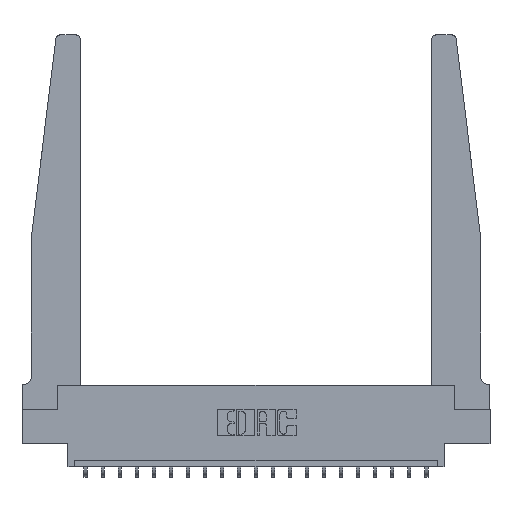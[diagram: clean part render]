
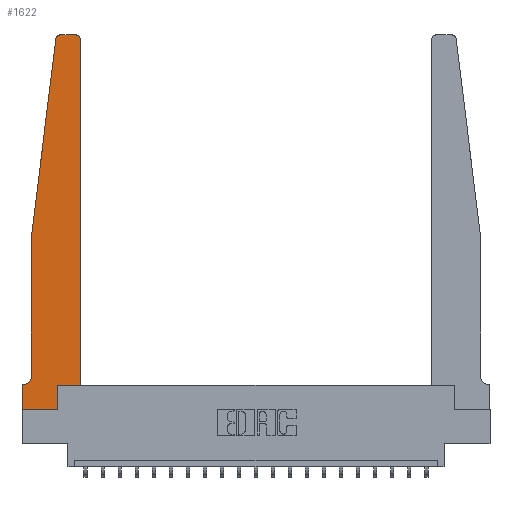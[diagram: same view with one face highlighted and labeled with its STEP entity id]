
A CAD part, top view. The second image highlights one B-rep face of the part: STEP entity #1622.
In plain terms, the highlighted planar face has unit normal (0, 0, 1).
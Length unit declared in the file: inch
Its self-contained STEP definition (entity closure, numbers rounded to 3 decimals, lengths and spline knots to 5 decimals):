
#86 = ORIENTED_EDGE ( 'NONE', *, *, #8515, .T. ) ;
#121 = CARTESIAN_POINT ( 'NONE',  ( 0., 0., 0.37 ) ) ;
#138 = ORIENTED_EDGE ( 'NONE', *, *, #15261, .T. ) ;
#257 = CARTESIAN_POINT ( 'NONE',  ( 0., 0., 0.37 ) ) ;
#797 = CARTESIAN_POINT ( 'NONE',  ( 0., 0., 0.37 ) ) ;
#815 = DIRECTION ( 'NONE',  ( -0.122, -0.992, 0. ) ) ;
#926 = CARTESIAN_POINT ( 'NONE',  ( 0.065, 1.25, 0.37 ) ) ;
#1312 = LINE ( 'NONE', #11413, #16584 ) ;
#1355 = VERTEX_POINT ( 'NONE', #17717 ) ;
#1390 = CARTESIAN_POINT ( 'NONE',  ( 0.015, 0.1875, 0.37 ) ) ;
#1622 = ADVANCED_FACE ( 'NONE', ( #16317 ), #19539, .T. ) ;
#1995 = VECTOR ( 'NONE', #9545, 39.37008 ) ;
#2030 = LINE ( 'NONE', #8608, #8117 ) ;
#2156 = VERTEX_POINT ( 'NONE', #10457 ) ;
#2339 = VERTEX_POINT ( 'NONE', #12402 ) ;
#2403 = EDGE_CURVE ( 'NONE', #16241, #1355, #1312, .T. ) ;
#2952 = EDGE_CURVE ( 'NONE', #19691, #5746, #2030, .T. ) ;
#3108 = VERTEX_POINT ( 'NONE', #16983 ) ;
#3351 = ORIENTED_EDGE ( 'NONE', *, *, #17008, .T. ) ;
#3553 = EDGE_CURVE ( 'NONE', #1355, #17381, #8109, .T. ) ;
#3592 = CARTESIAN_POINT ( 'NONE',  ( 0.27653, 2.75, 0.37 ) ) ;
#3903 = ORIENTED_EDGE ( 'NONE', *, *, #17429, .T. ) ;
#4144 = DIRECTION ( 'NONE',  ( 1., 0., 0. ) ) ;
#4485 = EDGE_CURVE ( 'NONE', #20452, #2156, #11691, .T. ) ;
#4582 = DIRECTION ( 'NONE',  ( 0., 0., -1. ) ) ;
#4667 = DIRECTION ( 'NONE',  ( 0., -1., 0. ) ) ;
#4692 = ORIENTED_EDGE ( 'NONE', *, *, #2403, .T. ) ;
#4798 = EDGE_CURVE ( 'NONE', #14378, #2339, #19421, .T. ) ;
#4809 = CARTESIAN_POINT ( 'NONE',  ( 0., 0.1875, 0.37 ) ) ;
#5261 = CARTESIAN_POINT ( 'NONE',  ( 0.2605, 0., 0.37 ) ) ;
#5374 = DIRECTION ( 'NONE',  ( 1., 0., 0. ) ) ;
#5746 = VERTEX_POINT ( 'NONE', #7887 ) ;
#7506 = LINE ( 'NONE', #926, #7927 ) ;
#7887 = CARTESIAN_POINT ( 'NONE',  ( 0.2605, 0.18, 0.37 ) ) ;
#7922 = CARTESIAN_POINT ( 'NONE',  ( 0.015, 0.2375, 0.37 ) ) ;
#7927 = VECTOR ( 'NONE', #815, 39.37008 ) ;
#8109 = LINE ( 'NONE', #121, #18549 ) ;
#8117 = VECTOR ( 'NONE', #8704, 39.37008 ) ;
#8212 = DIRECTION ( 'NONE',  ( -1., 0., 0. ) ) ;
#8515 = EDGE_CURVE ( 'NONE', #12634, #16777, #20770, .T. ) ;
#8608 = CARTESIAN_POINT ( 'NONE',  ( 0.2605, 0.18, 0.37 ) ) ;
#8704 = DIRECTION ( 'NONE',  ( 0., 1., 0. ) ) ;
#8767 = DIRECTION ( 'NONE',  ( 0., 0., 1. ) ) ;
#8903 = ORIENTED_EDGE ( 'NONE', *, *, #4798, .T. ) ;
#9539 = ORIENTED_EDGE ( 'NONE', *, *, #13835, .T. ) ;
#9545 = DIRECTION ( 'NONE',  ( 0., 1., 0. ) ) ;
#10457 = CARTESIAN_POINT ( 'NONE',  ( 0.065, 0.2375, 0.37 ) ) ;
#10660 = VECTOR ( 'NONE', #18340, 39.37008 ) ;
#11119 = DIRECTION ( 'NONE',  ( 0., 0., 1. ) ) ;
#11406 = CARTESIAN_POINT ( 'NONE',  ( 0.065, 1.25, 0.37 ) ) ;
#11413 = CARTESIAN_POINT ( 'NONE',  ( 0.065, 0.1875, 0.37 ) ) ;
#11642 = AXIS2_PLACEMENT_3D ( 'NONE', #12601, #21010, #19383 ) ;
#11691 = LINE ( 'NONE', #18465, #15013 ) ;
#11775 = LINE ( 'NONE', #17915, #10660 ) ;
#12402 = CARTESIAN_POINT ( 'NONE',  ( 0.425, 2.72, 0.37 ) ) ;
#12558 = CARTESIAN_POINT ( 'NONE',  ( 0.24675, 2.72367, 0.37 ) ) ;
#12600 = ORIENTED_EDGE ( 'NONE', *, *, #2952, .T. ) ;
#12601 = CARTESIAN_POINT ( 'NONE',  ( 0.395, 2.72, 0.37 ) ) ;
#12634 = VERTEX_POINT ( 'NONE', #3592 ) ;
#12652 = CIRCLE ( 'NONE', #17487, 0.05 ) ;
#12858 = CARTESIAN_POINT ( 'NONE',  ( 0.425, 0.18, 0.37 ) ) ;
#13240 = ORIENTED_EDGE ( 'NONE', *, *, #16314, .T. ) ;
#13732 = AXIS2_PLACEMENT_3D ( 'NONE', #4809, #8767, #18668 ) ;
#13835 = EDGE_CURVE ( 'NONE', #17381, #19691, #18769, .T. ) ;
#14378 = VERTEX_POINT ( 'NONE', #19277 ) ;
#15013 = VECTOR ( 'NONE', #19873, 39.37008 ) ;
#15261 = EDGE_CURVE ( 'NONE', #2156, #16241, #12652, .T. ) ;
#15637 = EDGE_CURVE ( 'NONE', #2339, #3108, #18181, .T. ) ;
#16073 = DIRECTION ( 'NONE',  ( -1., 0., 0. ) ) ;
#16241 = VERTEX_POINT ( 'NONE', #1390 ) ;
#16314 = EDGE_CURVE ( 'NONE', #5746, #14378, #20417, .T. ) ;
#16317 = FACE_OUTER_BOUND ( 'NONE', #19368, .T. ) ;
#16506 = CARTESIAN_POINT ( 'NONE',  ( 0.27653, 2.72, 0.37 ) ) ;
#16584 = VECTOR ( 'NONE', #8212, 39.37008 ) ;
#16772 = CARTESIAN_POINT ( 'NONE',  ( 0.425, 0.18, 0.37 ) ) ;
#16777 = VERTEX_POINT ( 'NONE', #12558 ) ;
#16983 = CARTESIAN_POINT ( 'NONE',  ( 0.395, 2.75, 0.37 ) ) ;
#17008 = EDGE_CURVE ( 'NONE', #16777, #20452, #7506, .T. ) ;
#17381 = VERTEX_POINT ( 'NONE', #257 ) ;
#17429 = EDGE_CURVE ( 'NONE', #3108, #12634, #11775, .T. ) ;
#17453 = ORIENTED_EDGE ( 'NONE', *, *, #4485, .T. ) ;
#17487 = AXIS2_PLACEMENT_3D ( 'NONE', #7922, #4582, #16073 ) ;
#17519 = VECTOR ( 'NONE', #5374, 39.37008 ) ;
#17717 = CARTESIAN_POINT ( 'NONE',  ( 0., 0.1875, 0.37 ) ) ;
#17915 = CARTESIAN_POINT ( 'NONE',  ( 0.25, 2.75, 0.37 ) ) ;
#18181 = CIRCLE ( 'NONE', #11642, 0.03 ) ;
#18340 = DIRECTION ( 'NONE',  ( -1., 0., 0. ) ) ;
#18465 = CARTESIAN_POINT ( 'NONE',  ( 0.065, 1.25, 0.37 ) ) ;
#18491 = ORIENTED_EDGE ( 'NONE', *, *, #3553, .T. ) ;
#18549 = VECTOR ( 'NONE', #4667, 39.37008 ) ;
#18668 = DIRECTION ( 'NONE',  ( 1., 0., 0. ) ) ;
#18769 = LINE ( 'NONE', #797, #20170 ) ;
#19277 = CARTESIAN_POINT ( 'NONE',  ( 0.425, 0.18, 0.37 ) ) ;
#19368 = EDGE_LOOP ( 'NONE', ( #3903, #86, #3351, #17453, #138, #4692, #18491, #9539, #12600, #13240, #8903, #20565 ) ) ;
#19383 = DIRECTION ( 'NONE',  ( 1., 0., 0. ) ) ;
#19421 = LINE ( 'NONE', #12858, #1995 ) ;
#19539 = PLANE ( 'NONE',  #13732 ) ;
#19691 = VERTEX_POINT ( 'NONE', #5261 ) ;
#19731 = DIRECTION ( 'NONE',  ( 1., 0., 0. ) ) ;
#19873 = DIRECTION ( 'NONE',  ( 0., -1., 0. ) ) ;
#20170 = VECTOR ( 'NONE', #4144, 39.37008 ) ;
#20417 = LINE ( 'NONE', #16772, #17519 ) ;
#20452 = VERTEX_POINT ( 'NONE', #11406 ) ;
#20565 = ORIENTED_EDGE ( 'NONE', *, *, #15637, .T. ) ;
#20770 = CIRCLE ( 'NONE', #21120, 0.03 ) ;
#21010 = DIRECTION ( 'NONE',  ( 0., 0., 1. ) ) ;
#21120 = AXIS2_PLACEMENT_3D ( 'NONE', #16506, #11119, #19731 ) ;
